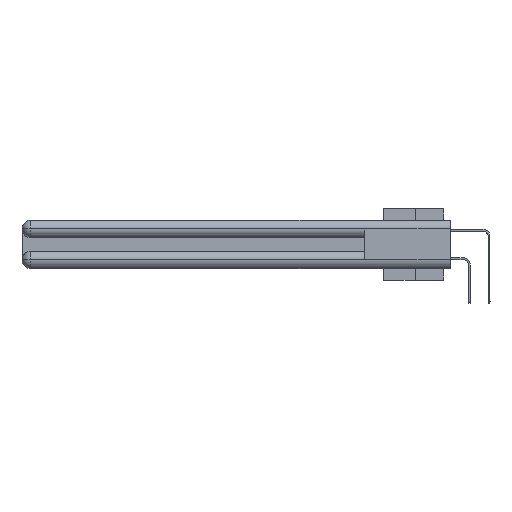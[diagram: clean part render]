
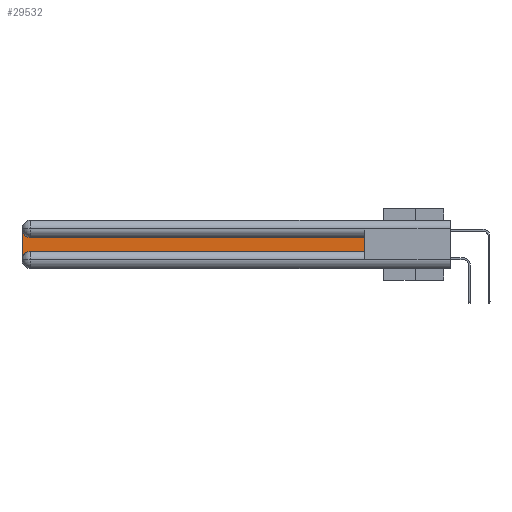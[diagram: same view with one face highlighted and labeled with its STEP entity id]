
A CAD part, left-side view. The second image highlights one B-rep face of the part: STEP entity #29532.
In plain terms, the highlighted planar face has unit normal (-1, 0, 0).
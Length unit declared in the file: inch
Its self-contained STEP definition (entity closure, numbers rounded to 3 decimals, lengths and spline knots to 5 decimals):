
#208 = ORIENTED_EDGE ( 'NONE', *, *, #31374, .T. ) ;
#297 = VECTOR ( 'NONE', #19146, 39.37008 ) ;
#356 = DIRECTION ( 'NONE',  ( 0., 1., 0. ) ) ;
#964 = AXIS2_PLACEMENT_3D ( 'NONE', #23037, #28138, #30357 ) ;
#1238 = ORIENTED_EDGE ( 'NONE', *, *, #1703, .T. ) ;
#1482 = LINE ( 'NONE', #23338, #297 ) ;
#1703 = EDGE_CURVE ( 'NONE', #14319, #23138, #24740, .T. ) ;
#2176 = FACE_OUTER_BOUND ( 'NONE', #26259, .T. ) ;
#2729 = CARTESIAN_POINT ( 'NONE',  ( 0.075, 0.6, -0.1225 ) ) ;
#4109 = DIRECTION ( 'NONE',  ( 0., 0., -1. ) ) ;
#4584 = CARTESIAN_POINT ( 'NONE',  ( 0.075, 2.94, -0.2775 ) ) ;
#6485 = AXIS2_PLACEMENT_3D ( 'NONE', #11916, #18626, #9052 ) ;
#6816 = LINE ( 'NONE', #28354, #15440 ) ;
#8364 = CIRCLE ( 'NONE', #20603, 0.06 ) ;
#9052 = DIRECTION ( 'NONE',  ( 0., 0., -1. ) ) ;
#9527 = PLANE ( 'NONE',  #6485 ) ;
#10538 = CARTESIAN_POINT ( 'NONE',  ( 0.075, 2.94, -0.1225 ) ) ;
#11916 = CARTESIAN_POINT ( 'NONE',  ( 0.075, 3., -0.1225 ) ) ;
#12057 = CARTESIAN_POINT ( 'NONE',  ( 0.075, 0.6, -0.1225 ) ) ;
#12106 = VECTOR ( 'NONE', #29551, 39.37008 ) ;
#12405 = ORIENTED_EDGE ( 'NONE', *, *, #23903, .T. ) ;
#12825 = CARTESIAN_POINT ( 'NONE',  ( 0.075, 3., -0.0625 ) ) ;
#14160 = DIRECTION ( 'NONE',  ( 1., 0., 0. ) ) ;
#14319 = VERTEX_POINT ( 'NONE', #12057 ) ;
#14737 = ORIENTED_EDGE ( 'NONE', *, *, #26011, .T. ) ;
#15186 = CARTESIAN_POINT ( 'NONE',  ( 0.075, 0.6, -0.2175 ) ) ;
#15440 = VECTOR ( 'NONE', #25792, 39.37008 ) ;
#15955 = VERTEX_POINT ( 'NONE', #25784 ) ;
#18626 = DIRECTION ( 'NONE',  ( 1., 0., 0. ) ) ;
#19146 = DIRECTION ( 'NONE',  ( 0., -1., 0. ) ) ;
#19498 = EDGE_CURVE ( 'NONE', #30412, #14319, #24003, .T. ) ;
#19904 = VECTOR ( 'NONE', #356, 39.37008 ) ;
#20603 = AXIS2_PLACEMENT_3D ( 'NONE', #4584, #14160, #4109 ) ;
#23037 = CARTESIAN_POINT ( 'NONE',  ( 0.075, 2.94, -0.0625 ) ) ;
#23138 = VERTEX_POINT ( 'NONE', #10538 ) ;
#23338 = CARTESIAN_POINT ( 'NONE',  ( 0.075, 0.6, -0.2175 ) ) ;
#23449 = ORIENTED_EDGE ( 'NONE', *, *, #19498, .T. ) ;
#23903 = EDGE_CURVE ( 'NONE', #25848, #15955, #6816, .T. ) ;
#24003 = LINE ( 'NONE', #29397, #12106 ) ;
#24740 = LINE ( 'NONE', #2729, #19904 ) ;
#25170 = EDGE_CURVE ( 'NONE', #15955, #31380, #8364, .T. ) ;
#25784 = CARTESIAN_POINT ( 'NONE',  ( 0.075, 3., -0.2775 ) ) ;
#25792 = DIRECTION ( 'NONE',  ( 0., 0., -1. ) ) ;
#25848 = VERTEX_POINT ( 'NONE', #12825 ) ;
#25924 = CIRCLE ( 'NONE', #964, 0.06 ) ;
#26011 = EDGE_CURVE ( 'NONE', #31380, #30412, #1482, .T. ) ;
#26259 = EDGE_LOOP ( 'NONE', ( #1238, #208, #12405, #29669, #14737, #23449 ) ) ;
#27970 = CARTESIAN_POINT ( 'NONE',  ( 0.075, 2.94, -0.2175 ) ) ;
#28138 = DIRECTION ( 'NONE',  ( 1., 0., 0. ) ) ;
#28354 = CARTESIAN_POINT ( 'NONE',  ( 0.075, 3., -0.2175 ) ) ;
#29397 = CARTESIAN_POINT ( 'NONE',  ( 0.075, 0.6, -0.2175 ) ) ;
#29532 = ADVANCED_FACE ( 'NONE', ( #2176 ), #9527, .F. ) ;
#29551 = DIRECTION ( 'NONE',  ( 0., 0., 1. ) ) ;
#29669 = ORIENTED_EDGE ( 'NONE', *, *, #25170, .T. ) ;
#30357 = DIRECTION ( 'NONE',  ( 0., 0., -1. ) ) ;
#30412 = VERTEX_POINT ( 'NONE', #15186 ) ;
#31374 = EDGE_CURVE ( 'NONE', #23138, #25848, #25924, .T. ) ;
#31380 = VERTEX_POINT ( 'NONE', #27970 ) ;
